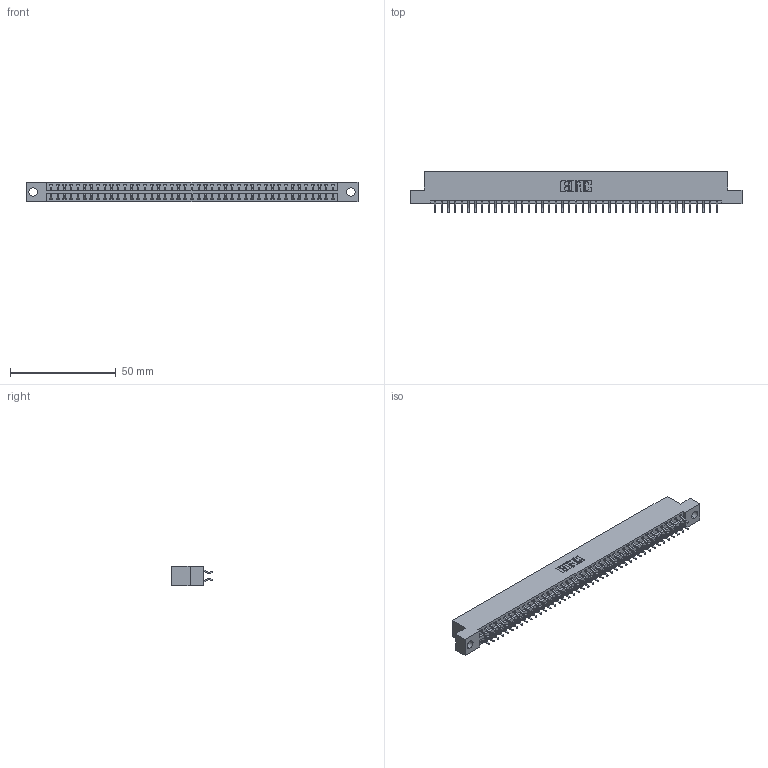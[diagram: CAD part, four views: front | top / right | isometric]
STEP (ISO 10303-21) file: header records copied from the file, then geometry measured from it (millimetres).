
FILE_DESCRIPTION (( 'STEP AP203' ), '1' );
FILE_NAME ('346-086-556-204.STEP', '2022-05-25T23:07:04', ( '' ), ( '' ), 'SwSTEP 2.0', 'SolidWorks 2020', '' );
FILE_SCHEMA (( 'CONFIG_CONTROL_DESIGN' ));
Length unit declared in the file: inch
Products named in the file (3): 345-292-001_556 Tail; 346-086-556-204; 346 Part_Flush Mounting Lugs - 0.156 Dia-TH
Assembly tree (87 placements, depth 2):
  346-086-556-204
    346 Part_Flush Mounting Lugs - 0.156 Dia-TH
    345-292-001_556 Tail  x86
Bounding box: 157.1 x 19.57 x 9.4 mm (x, y, z)
Volume: 15217.5 mm3; surface area: 20701.2 mm2
Topology: 87 solids, 87 shells, 5124 faces, 15243 edges, 10046 vertices
Faces by surface type: plane 3444, cylinder 1680
Entity records: 28567 total; most frequent: CARTESIAN_POINT 4726, ORIENTED_EDGE 4646, DIRECTION 4203, EDGE_CURVE 2323, LINE 2011, VECTOR 2011, VERTEX_POINT 1546, AXIS2_PLACEMENT_3D 1096
